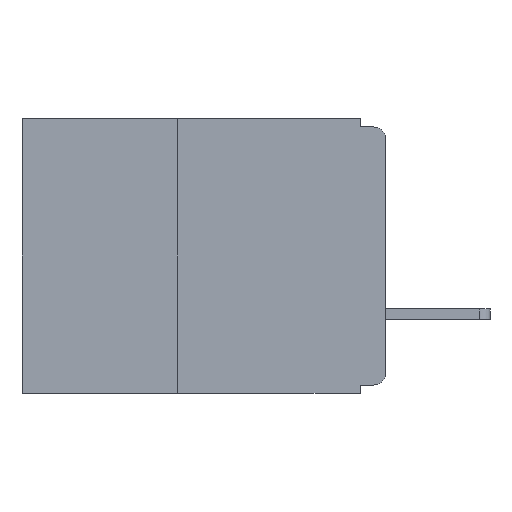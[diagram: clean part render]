
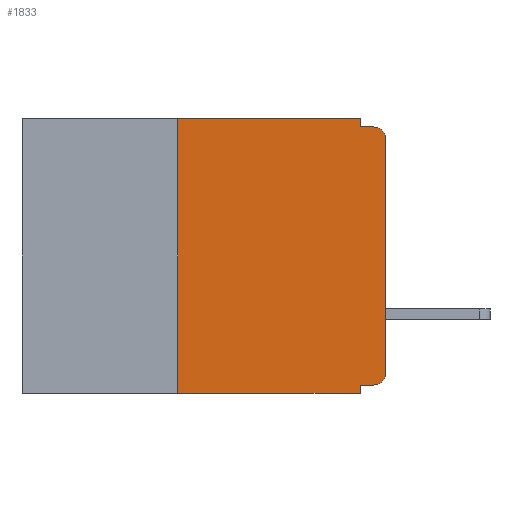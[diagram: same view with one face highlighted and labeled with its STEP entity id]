
A CAD part, left-side view. The second image highlights one B-rep face of the part: STEP entity #1833.
In plain terms, the highlighted planar face has unit normal (-1, 0, 0).
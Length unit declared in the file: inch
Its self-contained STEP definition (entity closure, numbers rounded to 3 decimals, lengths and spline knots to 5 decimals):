
#471 = CARTESIAN_POINT ( 'NONE',  ( 0., 0.437, 0. ) ) ;
#547 = VECTOR ( 'NONE', #7864, 39.37008 ) ;
#1092 = CARTESIAN_POINT ( 'NONE',  ( 0., 0.031, -0.32 ) ) ;
#1170 = ORIENTED_EDGE ( 'NONE', *, *, #17723, .T. ) ;
#1197 = VECTOR ( 'NONE', #8088, 39.37008 ) ;
#1833 = ADVANCED_FACE ( 'NONE', ( #2789 ), #13878, .F. ) ;
#1841 = VERTEX_POINT ( 'NONE', #19621 ) ;
#1880 = CARTESIAN_POINT ( 'NONE',  ( 0., 0.015, -0.025 ) ) ;
#2186 = ORIENTED_EDGE ( 'NONE', *, *, #9374, .T. ) ;
#2734 = ORIENTED_EDGE ( 'NONE', *, *, #4448, .F. ) ;
#2789 = FACE_OUTER_BOUND ( 'NONE', #7411, .T. ) ;
#2849 = CIRCLE ( 'NONE', #10973, 0.015 ) ;
#4013 = LINE ( 'NONE', #6763, #8764 ) ;
#4269 = CARTESIAN_POINT ( 'NONE',  ( 0., 0.031, -0.01 ) ) ;
#4278 = ORIENTED_EDGE ( 'NONE', *, *, #11505, .F. ) ;
#4448 = EDGE_CURVE ( 'NONE', #6193, #23784, #4013, .T. ) ;
#4514 = ORIENTED_EDGE ( 'NONE', *, *, #24383, .F. ) ;
#4901 = VERTEX_POINT ( 'NONE', #20763 ) ;
#5474 = CARTESIAN_POINT ( 'NONE',  ( 0., 0.015, -0.01 ) ) ;
#5505 = EDGE_CURVE ( 'NONE', #1841, #12369, #19745, .T. ) ;
#5801 = CARTESIAN_POINT ( 'NONE',  ( 0., 0.031, 0. ) ) ;
#5828 = EDGE_CURVE ( 'NONE', #1841, #8780, #6491, .T. ) ;
#5901 = EDGE_CURVE ( 'NONE', #4901, #7259, #17572, .T. ) ;
#6193 = VERTEX_POINT ( 'NONE', #4269 ) ;
#6397 = CARTESIAN_POINT ( 'NONE',  ( 0., 0., -0.025 ) ) ;
#6411 = DIRECTION ( 'NONE',  ( 0., -1., 0. ) ) ;
#6491 = LINE ( 'NONE', #8246, #1197 ) ;
#6763 = CARTESIAN_POINT ( 'NONE',  ( 0., 0., -0.01 ) ) ;
#7036 = DIRECTION ( 'NONE',  ( 0., -1., 0. ) ) ;
#7259 = VERTEX_POINT ( 'NONE', #1092 ) ;
#7389 = VERTEX_POINT ( 'NONE', #24143 ) ;
#7390 = CARTESIAN_POINT ( 'NONE',  ( 0., 0., -0.32 ) ) ;
#7411 = EDGE_LOOP ( 'NONE', ( #1170, #2186, #2734, #4278, #4514, #8642, #11906, #12123, #16119, #17473 ) ) ;
#7831 = CARTESIAN_POINT ( 'NONE',  ( 0., 0.25, 0. ) ) ;
#7864 = DIRECTION ( 'NONE',  ( 0., 1., 0. ) ) ;
#7953 = EDGE_CURVE ( 'NONE', #7259, #12369, #21146, .T. ) ;
#8088 = DIRECTION ( 'NONE',  ( 0., 0., 1. ) ) ;
#8246 = CARTESIAN_POINT ( 'NONE',  ( 0., 0.25, -0.33 ) ) ;
#8642 = ORIENTED_EDGE ( 'NONE', *, *, #5828, .F. ) ;
#8764 = VECTOR ( 'NONE', #7036, 39.37008 ) ;
#8780 = VERTEX_POINT ( 'NONE', #7831 ) ;
#9143 = CARTESIAN_POINT ( 'NONE',  ( 0., 0.015, -0.305 ) ) ;
#9374 = EDGE_CURVE ( 'NONE', #18557, #23784, #2849, .T. ) ;
#9764 = CIRCLE ( 'NONE', #23940, 0.015 ) ;
#9910 = CARTESIAN_POINT ( 'NONE',  ( 0., 0., 0. ) ) ;
#10973 = AXIS2_PLACEMENT_3D ( 'NONE', #1880, #15033, #23664 ) ;
#11064 = DIRECTION ( 'NONE',  ( 0., 0., -1. ) ) ;
#11505 = EDGE_CURVE ( 'NONE', #14450, #6193, #25270, .T. ) ;
#11906 = ORIENTED_EDGE ( 'NONE', *, *, #5505, .T. ) ;
#12123 = ORIENTED_EDGE ( 'NONE', *, *, #7953, .F. ) ;
#12162 = DIRECTION ( 'NONE',  ( 0., -1., 0. ) ) ;
#12224 = CARTESIAN_POINT ( 'NONE',  ( 0., 0.437, -0.33 ) ) ;
#12369 = VERTEX_POINT ( 'NONE', #20005 ) ;
#13806 = DIRECTION ( 'NONE',  ( 0., 0., 1. ) ) ;
#13878 = PLANE ( 'NONE',  #25005 ) ;
#13922 = VECTOR ( 'NONE', #12162, 39.37008 ) ;
#14450 = VERTEX_POINT ( 'NONE', #5801 ) ;
#15033 = DIRECTION ( 'NONE',  ( -1., 0., 0. ) ) ;
#15397 = CARTESIAN_POINT ( 'NONE',  ( 0., 0.031, 0. ) ) ;
#16119 = ORIENTED_EDGE ( 'NONE', *, *, #5901, .F. ) ;
#16626 = DIRECTION ( 'NONE',  ( 1., 0., 0. ) ) ;
#17473 = ORIENTED_EDGE ( 'NONE', *, *, #21951, .T. ) ;
#17572 = LINE ( 'NONE', #7390, #547 ) ;
#17579 = DIRECTION ( 'NONE',  ( 0., 0., -1. ) ) ;
#17656 = CARTESIAN_POINT ( 'NONE',  ( 0., 0.031, -0.33 ) ) ;
#17723 = EDGE_CURVE ( 'NONE', #7389, #18557, #19587, .T. ) ;
#18557 = VERTEX_POINT ( 'NONE', #6397 ) ;
#19567 = VECTOR ( 'NONE', #21328, 39.37008 ) ;
#19587 = LINE ( 'NONE', #9910, #24128 ) ;
#19621 = CARTESIAN_POINT ( 'NONE',  ( 0., 0.25, -0.33 ) ) ;
#19745 = LINE ( 'NONE', #12224, #13922 ) ;
#20005 = CARTESIAN_POINT ( 'NONE',  ( 0., 0.031, -0.33 ) ) ;
#20526 = VECTOR ( 'NONE', #17579, 39.37008 ) ;
#20763 = CARTESIAN_POINT ( 'NONE',  ( 0., 0.015, -0.32 ) ) ;
#21146 = LINE ( 'NONE', #17656, #20526 ) ;
#21328 = DIRECTION ( 'NONE',  ( 0., 0., -1. ) ) ;
#21951 = EDGE_CURVE ( 'NONE', #4901, #7389, #9764, .T. ) ;
#22782 = DIRECTION ( 'NONE',  ( -1., 0., 0. ) ) ;
#23071 = CARTESIAN_POINT ( 'NONE',  ( 0., 0.437, 0. ) ) ;
#23664 = DIRECTION ( 'NONE',  ( 0., 0., -1. ) ) ;
#23784 = VERTEX_POINT ( 'NONE', #5474 ) ;
#23940 = AXIS2_PLACEMENT_3D ( 'NONE', #9143, #22782, #11064 ) ;
#24128 = VECTOR ( 'NONE', #13806, 39.37008 ) ;
#24143 = CARTESIAN_POINT ( 'NONE',  ( 0., 0., -0.305 ) ) ;
#24219 = VECTOR ( 'NONE', #6411, 39.37008 ) ;
#24383 = EDGE_CURVE ( 'NONE', #8780, #14450, #24792, .T. ) ;
#24789 = DIRECTION ( 'NONE',  ( 0., 0., -1. ) ) ;
#24792 = LINE ( 'NONE', #471, #24219 ) ;
#25005 = AXIS2_PLACEMENT_3D ( 'NONE', #23071, #16626, #24789 ) ;
#25270 = LINE ( 'NONE', #15397, #19567 ) ;
